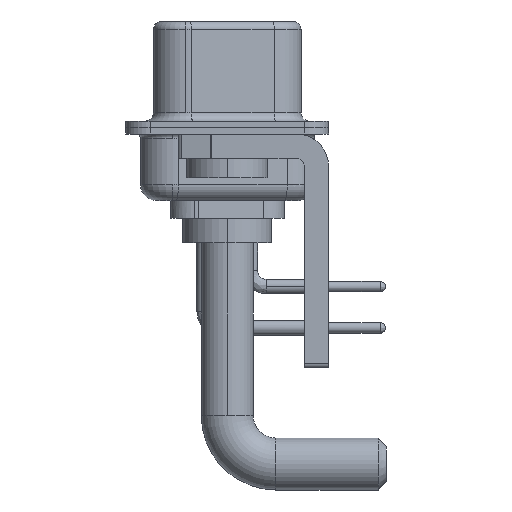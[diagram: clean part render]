
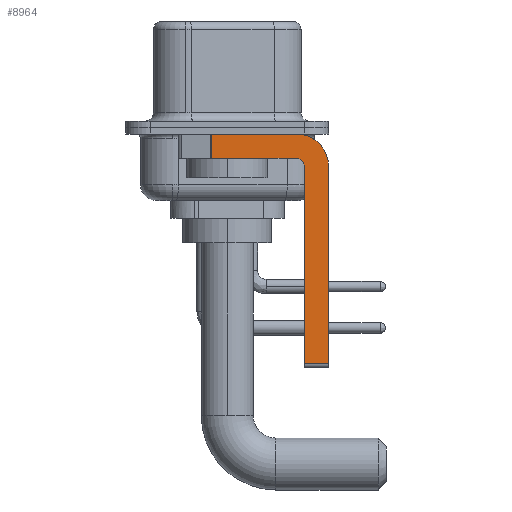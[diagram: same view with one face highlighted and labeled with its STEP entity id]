
A CAD part, left-side view. The second image highlights one B-rep face of the part: STEP entity #8964.
In plain terms, the highlighted planar face has unit normal (-1, 0, 0).
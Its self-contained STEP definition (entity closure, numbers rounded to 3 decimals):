
#850 = VECTOR ( 'NONE', #16926, 1000. ) ;
#1340 = EDGE_CURVE ( 'NONE', #16939, #7997, #10347, .T. ) ;
#1345 = CARTESIAN_POINT ( 'NONE',  ( -2.9, -4.25, -0.4 ) ) ;
#2367 = DIRECTION ( 'NONE',  ( 0., 0., -1. ) ) ;
#2786 = VECTOR ( 'NONE', #14625, 1000. ) ;
#3526 = CARTESIAN_POINT ( 'NONE',  ( -2.9, 0.978, -1.9 ) ) ;
#4021 = EDGE_CURVE ( 'NONE', #16939, #19627, #26468, .T. ) ;
#4038 = DIRECTION ( 'NONE',  ( 1., 0., 0. ) ) ;
#5820 = CARTESIAN_POINT ( 'NONE',  ( -2.9, -6.25, -2.4 ) ) ;
#6020 = VECTOR ( 'NONE', #15125, 1000. ) ;
#6237 = EDGE_CURVE ( 'NONE', #6821, #19627, #23707, .T. ) ;
#6317 = VECTOR ( 'NONE', #2367, 1000. ) ;
#6609 = CIRCLE ( 'NONE', #8035, 2. ) ;
#6821 = VERTEX_POINT ( 'NONE', #29318 ) ;
#6868 = DIRECTION ( 'NONE',  ( 0., 0., -1. ) ) ;
#7137 = ORIENTED_EDGE ( 'NONE', *, *, #4021, .T. ) ;
#7519 = DIRECTION ( 'NONE',  ( 0., 0., 1. ) ) ;
#7527 = AXIS2_PLACEMENT_3D ( 'NONE', #15199, #21620, #7913 ) ;
#7913 = DIRECTION ( 'NONE',  ( 0., 0., 1. ) ) ;
#7997 = VERTEX_POINT ( 'NONE', #1345 ) ;
#8035 = AXIS2_PLACEMENT_3D ( 'NONE', #25030, #4038, #6868 ) ;
#8507 = DIRECTION ( 'NONE',  ( 0., 0., -1. ) ) ;
#8628 = ORIENTED_EDGE ( 'NONE', *, *, #21528, .F. ) ;
#8964 = ADVANCED_FACE ( 'NONE', ( #10746 ), #19834, .F. ) ;
#9109 = ORIENTED_EDGE ( 'NONE', *, *, #25292, .F. ) ;
#9214 = CARTESIAN_POINT ( 'NONE',  ( -2.9, -6.25, -2.4 ) ) ;
#9624 = CARTESIAN_POINT ( 'NONE',  ( -2.9, -4.25, -14.55 ) ) ;
#10347 = LINE ( 'NONE', #28574, #27788 ) ;
#10431 = EDGE_LOOP ( 'NONE', ( #15055, #7137, #14214, #9109, #8628, #13224, #13640, #27497 ) ) ;
#10746 = FACE_OUTER_BOUND ( 'NONE', #10431, .T. ) ;
#11742 = LINE ( 'NONE', #9214, #6317 ) ;
#11838 = LINE ( 'NONE', #16172, #17637 ) ;
#12510 = CARTESIAN_POINT ( 'NONE',  ( -2.9, 0.978, -1.9 ) ) ;
#13224 = ORIENTED_EDGE ( 'NONE', *, *, #17065, .T. ) ;
#13640 = ORIENTED_EDGE ( 'NONE', *, *, #24565, .F. ) ;
#14059 = CARTESIAN_POINT ( 'NONE',  ( -2.9, -4.75, -2.4 ) ) ;
#14214 = ORIENTED_EDGE ( 'NONE', *, *, #6237, .F. ) ;
#14625 = DIRECTION ( 'NONE',  ( 0., 1., 0. ) ) ;
#14746 = AXIS2_PLACEMENT_3D ( 'NONE', #26707, #28958, #8507 ) ;
#15055 = ORIENTED_EDGE ( 'NONE', *, *, #1340, .F. ) ;
#15125 = DIRECTION ( 'NONE',  ( 0., 0., -1. ) ) ;
#15199 = CARTESIAN_POINT ( 'NONE',  ( -2.9, -4.25, -2.4 ) ) ;
#16172 = CARTESIAN_POINT ( 'NONE',  ( -2.9, -4.75, -14.8 ) ) ;
#16926 = DIRECTION ( 'NONE',  ( 0., -1., 0. ) ) ;
#16939 = VERTEX_POINT ( 'NONE', #23628 ) ;
#17065 = EDGE_CURVE ( 'NONE', #19949, #19846, #23487, .T. ) ;
#17637 = VECTOR ( 'NONE', #7519, 1000. ) ;
#19318 = EDGE_CURVE ( 'NONE', #7997, #27939, #6609, .T. ) ;
#19627 = VERTEX_POINT ( 'NONE', #12510 ) ;
#19834 = PLANE ( 'NONE',  #14746 ) ;
#19846 = VERTEX_POINT ( 'NONE', #20505 ) ;
#19949 = VERTEX_POINT ( 'NONE', #26028 ) ;
#20505 = CARTESIAN_POINT ( 'NONE',  ( -2.9, -6.25, -14.55 ) ) ;
#21528 = EDGE_CURVE ( 'NONE', #19949, #25508, #11838, .T. ) ;
#21620 = DIRECTION ( 'NONE',  ( -1., 0., 0. ) ) ;
#23487 = LINE ( 'NONE', #9624, #850 ) ;
#23628 = CARTESIAN_POINT ( 'NONE',  ( -2.9, 0.978, -0.4 ) ) ;
#23707 = LINE ( 'NONE', #26265, #2786 ) ;
#24357 = DIRECTION ( 'NONE',  ( 0., -1., 0. ) ) ;
#24565 = EDGE_CURVE ( 'NONE', #27939, #19846, #11742, .T. ) ;
#25030 = CARTESIAN_POINT ( 'NONE',  ( -2.9, -4.25, -2.4 ) ) ;
#25292 = EDGE_CURVE ( 'NONE', #25508, #6821, #27035, .T. ) ;
#25508 = VERTEX_POINT ( 'NONE', #14059 ) ;
#26028 = CARTESIAN_POINT ( 'NONE',  ( -2.9, -4.75, -14.55 ) ) ;
#26265 = CARTESIAN_POINT ( 'NONE',  ( -2.9, -4.25, -1.9 ) ) ;
#26468 = LINE ( 'NONE', #3526, #6020 ) ;
#26707 = CARTESIAN_POINT ( 'NONE',  ( -2.9, -4.25, -2.4 ) ) ;
#27035 = CIRCLE ( 'NONE', #7527, 0.5 ) ;
#27497 = ORIENTED_EDGE ( 'NONE', *, *, #19318, .F. ) ;
#27788 = VECTOR ( 'NONE', #24357, 1000. ) ;
#27939 = VERTEX_POINT ( 'NONE', #5820 ) ;
#28574 = CARTESIAN_POINT ( 'NONE',  ( -2.9, 3., -0.4 ) ) ;
#28958 = DIRECTION ( 'NONE',  ( 1., 0., 0. ) ) ;
#29318 = CARTESIAN_POINT ( 'NONE',  ( -2.9, -4.25, -1.9 ) ) ;
